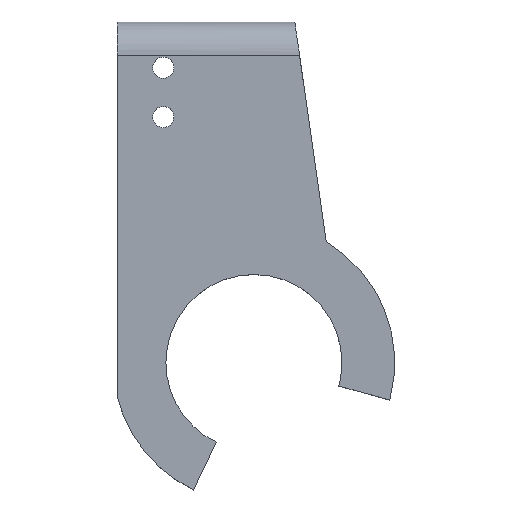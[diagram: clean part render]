
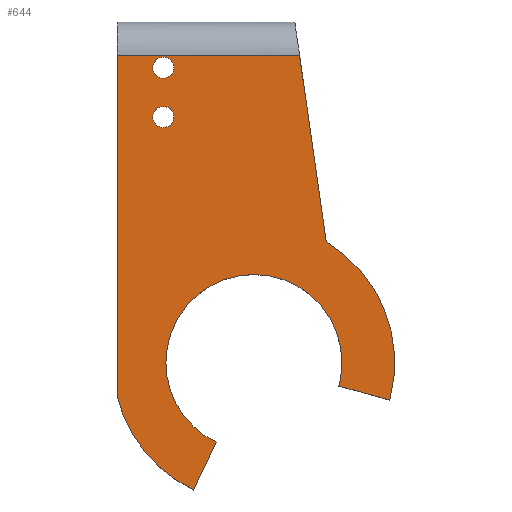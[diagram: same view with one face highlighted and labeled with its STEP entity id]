
A CAD part, top view. The second image highlights one B-rep face of the part: STEP entity #644.
In plain terms, the highlighted planar face has unit normal (0, 0, 1).
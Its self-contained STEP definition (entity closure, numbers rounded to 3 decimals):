
#12 = VERTEX_POINT ( 'NONE', #567 ) ;
#13 = EDGE_CURVE ( 'NONE', #42, #620, #158, .T. ) ;
#17 = CARTESIAN_POINT ( 'NONE',  ( 50.742, -83.726, 15. ) ) ;
#19 = DIRECTION ( 'NONE',  ( 1., 0., 0. ) ) ;
#25 = CARTESIAN_POINT ( 'NONE',  ( 25.742, -83.726, 15. ) ) ;
#30 = VERTEX_POINT ( 'NONE', #493 ) ;
#34 = EDGE_CURVE ( 'NONE', #472, #736, #504, .T. ) ;
#42 = VERTEX_POINT ( 'NONE', #164 ) ;
#53 = DIRECTION ( 'NONE',  ( 0., 0., -1. ) ) ;
#62 = LINE ( 'NONE', #713, #525 ) ;
#68 = AXIS2_PLACEMENT_3D ( 'NONE', #426, #574, #498 ) ;
#86 = DIRECTION ( 'NONE',  ( 1., 0., 0. ) ) ;
#87 = LINE ( 'NONE', #358, #616 ) ;
#110 = AXIS2_PLACEMENT_3D ( 'NONE', #677, #484, #19 ) ;
#127 = EDGE_CURVE ( 'NONE', #30, #472, #666, .T. ) ;
#133 = ORIENTED_EDGE ( 'NONE', *, *, #827, .T. ) ;
#136 = CARTESIAN_POINT ( 'NONE',  ( -13., 13., 15. ) ) ;
#143 = CARTESIAN_POINT ( 'NONE',  ( 49.841, -90.377, 15. ) ) ;
#158 = CIRCLE ( 'NONE', #384, 3. ) ;
#163 = EDGE_CURVE ( 'NONE', #445, #30, #727, .T. ) ;
#164 = CARTESIAN_POINT ( 'NONE',  ( -3., 0., 15. ) ) ;
#166 = AXIS2_PLACEMENT_3D ( 'NONE', #627, #495, #760 ) ;
#173 = CARTESIAN_POINT ( 'NONE',  ( 0., 0., 15. ) ) ;
#185 = VERTEX_POINT ( 'NONE', #737 ) ;
#200 = VERTEX_POINT ( 'NONE', #609 ) ;
#201 = VERTEX_POINT ( 'NONE', #17 ) ;
#203 = CIRCLE ( 'NONE', #333, 3. ) ;
#204 = ORIENTED_EDGE ( 'NONE', *, *, #778, .T. ) ;
#209 = CARTESIAN_POINT ( 'NONE',  ( 25.742, 3.5, 15. ) ) ;
#223 = DIRECTION ( 'NONE',  ( 1., 0., 0. ) ) ;
#239 = CARTESIAN_POINT ( 'NONE',  ( -3., -14., 15. ) ) ;
#242 = EDGE_CURVE ( 'NONE', #200, #398, #401, .T. ) ;
#250 = DIRECTION ( 'NONE',  ( 0., 0., -1. ) ) ;
#254 = AXIS2_PLACEMENT_3D ( 'NONE', #25, #424, #355 ) ;
#257 = CARTESIAN_POINT ( 'NONE',  ( 49.841, -90.377, 15. ) ) ;
#258 = ORIENTED_EDGE ( 'NONE', *, *, #466, .T. ) ;
#260 = CIRCLE ( 'NONE', #794, 3. ) ;
#273 = LINE ( 'NONE', #143, #702 ) ;
#288 = DIRECTION ( 'NONE',  ( 0., -1., 0. ) ) ;
#289 = DIRECTION ( 'NONE',  ( 0., 0., 1. ) ) ;
#290 = EDGE_CURVE ( 'NONE', #531, #502, #622, .T. ) ;
#291 = AXIS2_PLACEMENT_3D ( 'NONE', #840, #250, #516 ) ;
#298 = ORIENTED_EDGE ( 'NONE', *, *, #13, .F. ) ;
#300 = VECTOR ( 'NONE', #477, 1000. ) ;
#303 = ORIENTED_EDGE ( 'NONE', *, *, #242, .F. ) ;
#310 = EDGE_CURVE ( 'NONE', #620, #42, #260, .T. ) ;
#318 = CARTESIAN_POINT ( 'NONE',  ( 3., 0., 15. ) ) ;
#333 = AXIS2_PLACEMENT_3D ( 'NONE', #473, #543, #86 ) ;
#344 = CIRCLE ( 'NONE', #483, 40. ) ;
#353 = EDGE_CURVE ( 'NONE', #185, #445, #87, .T. ) ;
#355 = DIRECTION ( 'NONE',  ( -1., 0., 0. ) ) ;
#358 = CARTESIAN_POINT ( 'NONE',  ( 46.289, -49.407, 15. ) ) ;
#364 = EDGE_LOOP ( 'NONE', ( #298, #665 ) ) ;
#384 = AXIS2_PLACEMENT_3D ( 'NONE', #173, #818, #829 ) ;
#386 = CARTESIAN_POINT ( 'NONE',  ( 8.635, -119.883, 15. ) ) ;
#398 = VERTEX_POINT ( 'NONE', #239 ) ;
#401 = CIRCLE ( 'NONE', #110, 3. ) ;
#404 = CARTESIAN_POINT ( 'NONE',  ( 0.742, -83.726, 15. ) ) ;
#422 = ORIENTED_EDGE ( 'NONE', *, *, #353, .T. ) ;
#424 = DIRECTION ( 'NONE',  ( 0., 0., -1. ) ) ;
#426 = CARTESIAN_POINT ( 'NONE',  ( 25.742, -83.726, 15. ) ) ;
#445 = VERTEX_POINT ( 'NONE', #576 ) ;
#458 = EDGE_CURVE ( 'NONE', #201, #795, #465, .T. ) ;
#465 = CIRCLE ( 'NONE', #291, 25. ) ;
#466 = EDGE_CURVE ( 'NONE', #12, #185, #344, .T. ) ;
#467 = CARTESIAN_POINT ( 'NONE',  ( 15.05, -106.324, 15. ) ) ;
#470 = ORIENTED_EDGE ( 'NONE', *, *, #34, .T. ) ;
#472 = VERTEX_POINT ( 'NONE', #723 ) ;
#473 = CARTESIAN_POINT ( 'NONE',  ( 0., -14., 15. ) ) ;
#476 = EDGE_LOOP ( 'NONE', ( #422, #556, #854, #470, #133, #580, #204, #552, #802, #258 ) ) ;
#477 = DIRECTION ( 'NONE',  ( -1., 0., 0. ) ) ;
#483 = AXIS2_PLACEMENT_3D ( 'NONE', #641, #657, #652 ) ;
#484 = DIRECTION ( 'NONE',  ( 0., 0., 1. ) ) ;
#493 = CARTESIAN_POINT ( 'NONE',  ( -13., 3.5, 15. ) ) ;
#495 = DIRECTION ( 'NONE',  ( 0., 0., -1. ) ) ;
#498 = DIRECTION ( 'NONE',  ( 1., 0., 0. ) ) ;
#500 = PLANE ( 'NONE',  #166 ) ;
#502 = VERTEX_POINT ( 'NONE', #404 ) ;
#504 = CIRCLE ( 'NONE', #68, 40. ) ;
#516 = DIRECTION ( 'NONE',  ( -1., 0., 0. ) ) ;
#521 = EDGE_CURVE ( 'NONE', #795, #12, #273, .T. ) ;
#522 = EDGE_CURVE ( 'NONE', #398, #200, #203, .T. ) ;
#525 = VECTOR ( 'NONE', #791, 1000. ) ;
#531 = VERTEX_POINT ( 'NONE', #467 ) ;
#543 = DIRECTION ( 'NONE',  ( 0., 0., 1. ) ) ;
#552 = ORIENTED_EDGE ( 'NONE', *, *, #458, .T. ) ;
#556 = ORIENTED_EDGE ( 'NONE', *, *, #163, .T. ) ;
#567 = CARTESIAN_POINT ( 'NONE',  ( 64.3, -94.368, 15. ) ) ;
#574 = DIRECTION ( 'NONE',  ( 0., 0., 1. ) ) ;
#576 = CARTESIAN_POINT ( 'NONE',  ( 38.706, 3.5, 15. ) ) ;
#580 = ORIENTED_EDGE ( 'NONE', *, *, #290, .T. ) ;
#599 = EDGE_LOOP ( 'NONE', ( #821, #303 ) ) ;
#600 = DIRECTION ( 'NONE',  ( 0.964, -0.266, 0. ) ) ;
#609 = CARTESIAN_POINT ( 'NONE',  ( 3., -14., 15. ) ) ;
#612 = CARTESIAN_POINT ( 'NONE',  ( 0., 0., 15. ) ) ;
#616 = VECTOR ( 'NONE', #617, 1000. ) ;
#617 = DIRECTION ( 'NONE',  ( -0.142, 0.99, 0. ) ) ;
#620 = VERTEX_POINT ( 'NONE', #318 ) ;
#622 = CIRCLE ( 'NONE', #254, 25. ) ;
#627 = CARTESIAN_POINT ( 'NONE',  ( 25.742, -83.726, 15. ) ) ;
#632 = FACE_OUTER_BOUND ( 'NONE', #476, .T. ) ;
#641 = CARTESIAN_POINT ( 'NONE',  ( 25.742, -83.726, 15. ) ) ;
#644 = ADVANCED_FACE ( 'NONE', ( #632, #688, #692 ), #500, .F. ) ;
#647 = CARTESIAN_POINT ( 'NONE',  ( 25.742, -83.726, 15. ) ) ;
#652 = DIRECTION ( 'NONE',  ( 1., 0., 0. ) ) ;
#657 = DIRECTION ( 'NONE',  ( 0., 0., 1. ) ) ;
#665 = ORIENTED_EDGE ( 'NONE', *, *, #310, .F. ) ;
#666 = LINE ( 'NONE', #136, #751 ) ;
#677 = CARTESIAN_POINT ( 'NONE',  ( 0., -14., 15. ) ) ;
#688 = FACE_BOUND ( 'NONE', #364, .T. ) ;
#692 = FACE_BOUND ( 'NONE', #599, .T. ) ;
#702 = VECTOR ( 'NONE', #600, 1000. ) ;
#713 = CARTESIAN_POINT ( 'NONE',  ( 8.635, -119.883, 15. ) ) ;
#723 = CARTESIAN_POINT ( 'NONE',  ( -13., -93.679, 15. ) ) ;
#727 = LINE ( 'NONE', #209, #300 ) ;
#736 = VERTEX_POINT ( 'NONE', #386 ) ;
#737 = CARTESIAN_POINT ( 'NONE',  ( 46.289, -49.407, 15. ) ) ;
#751 = VECTOR ( 'NONE', #288, 1000. ) ;
#760 = DIRECTION ( 'NONE',  ( -1., 0., 0. ) ) ;
#778 = EDGE_CURVE ( 'NONE', #502, #201, #828, .T. ) ;
#791 = DIRECTION ( 'NONE',  ( 0.428, 0.904, 0. ) ) ;
#794 = AXIS2_PLACEMENT_3D ( 'NONE', #612, #289, #223 ) ;
#795 = VERTEX_POINT ( 'NONE', #257 ) ;
#796 = AXIS2_PLACEMENT_3D ( 'NONE', #647, #53, #847 ) ;
#802 = ORIENTED_EDGE ( 'NONE', *, *, #521, .T. ) ;
#818 = DIRECTION ( 'NONE',  ( 0., 0., 1. ) ) ;
#821 = ORIENTED_EDGE ( 'NONE', *, *, #522, .F. ) ;
#827 = EDGE_CURVE ( 'NONE', #736, #531, #62, .T. ) ;
#828 = CIRCLE ( 'NONE', #796, 25. ) ;
#829 = DIRECTION ( 'NONE',  ( 1., 0., 0. ) ) ;
#840 = CARTESIAN_POINT ( 'NONE',  ( 25.742, -83.726, 15. ) ) ;
#847 = DIRECTION ( 'NONE',  ( -1., 0., 0. ) ) ;
#854 = ORIENTED_EDGE ( 'NONE', *, *, #127, .T. ) ;
